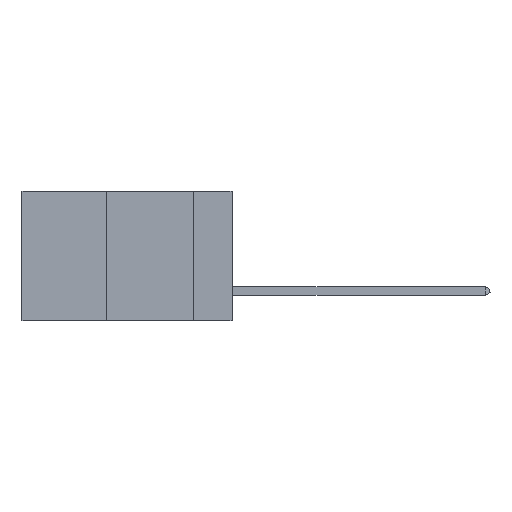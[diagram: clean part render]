
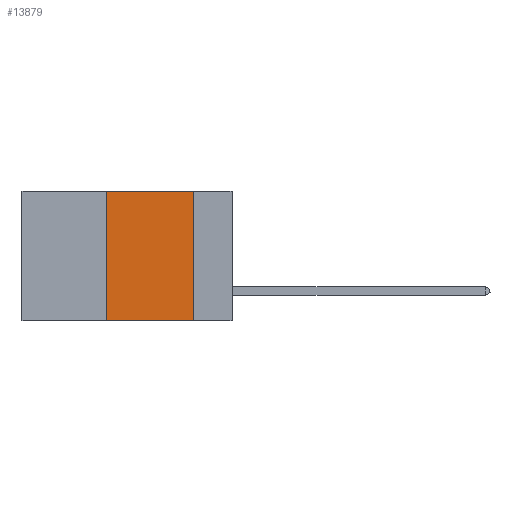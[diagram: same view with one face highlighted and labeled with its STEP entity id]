
A CAD part, left-side view. The second image highlights one B-rep face of the part: STEP entity #13879.
In plain terms, the highlighted planar face has unit normal (-1, 0, 0).
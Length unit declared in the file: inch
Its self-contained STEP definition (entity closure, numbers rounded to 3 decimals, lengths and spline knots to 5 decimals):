
#1645 = EDGE_LOOP ( 'NONE', ( #18609, #4746, #25784, #2938 ) ) ;
#2938 = ORIENTED_EDGE ( 'NONE', *, *, #21262, .T. ) ;
#3064 = DIRECTION ( 'NONE',  ( 0., 0., -1. ) ) ;
#3400 = CARTESIAN_POINT ( 'NONE',  ( 0., 0.36, 0. ) ) ;
#4480 = CARTESIAN_POINT ( 'NONE',  ( 0., 0.6, 0. ) ) ;
#4516 = CARTESIAN_POINT ( 'NONE',  ( 0., 0.11, -0.37 ) ) ;
#4746 = ORIENTED_EDGE ( 'NONE', *, *, #12196, .F. ) ;
#4916 = DIRECTION ( 'NONE',  ( 0., -1., 0. ) ) ;
#5689 = EDGE_CURVE ( 'NONE', #15217, #21051, #22135, .T. ) ;
#6246 = VECTOR ( 'NONE', #3064, 39.37008 ) ;
#6550 = CARTESIAN_POINT ( 'NONE',  ( 0., 0.6, 0. ) ) ;
#6699 = LINE ( 'NONE', #25753, #9295 ) ;
#7883 = EDGE_CURVE ( 'NONE', #17544, #24562, #24001, .T. ) ;
#8630 = DIRECTION ( 'NONE',  ( 0., 0., -1. ) ) ;
#9295 = VECTOR ( 'NONE', #17797, 39.37008 ) ;
#12196 = EDGE_CURVE ( 'NONE', #24562, #15217, #14061, .T. ) ;
#13486 = CARTESIAN_POINT ( 'NONE',  ( 0., 0.11, 0. ) ) ;
#13879 = ADVANCED_FACE ( 'NONE', ( #23405 ), #25015, .F. ) ;
#14061 = LINE ( 'NONE', #4480, #25749 ) ;
#15217 = VERTEX_POINT ( 'NONE', #22149 ) ;
#16197 = AXIS2_PLACEMENT_3D ( 'NONE', #6550, #21054, #8630 ) ;
#16597 = DIRECTION ( 'NONE',  ( 0., 0., 1. ) ) ;
#17526 = CARTESIAN_POINT ( 'NONE',  ( 0., 0.36, -0.37 ) ) ;
#17544 = VERTEX_POINT ( 'NONE', #17526 ) ;
#17797 = DIRECTION ( 'NONE',  ( 0., -1., 0. ) ) ;
#18581 = CARTESIAN_POINT ( 'NONE',  ( 0., 0.36, 0. ) ) ;
#18609 = ORIENTED_EDGE ( 'NONE', *, *, #5689, .F. ) ;
#21051 = VERTEX_POINT ( 'NONE', #4516 ) ;
#21054 = DIRECTION ( 'NONE',  ( 1., 0., 0. ) ) ;
#21262 = EDGE_CURVE ( 'NONE', #17544, #21051, #6699, .T. ) ;
#22135 = LINE ( 'NONE', #13486, #6246 ) ;
#22149 = CARTESIAN_POINT ( 'NONE',  ( 0., 0.11, 0. ) ) ;
#22372 = VECTOR ( 'NONE', #16597, 39.37008 ) ;
#23405 = FACE_OUTER_BOUND ( 'NONE', #1645, .T. ) ;
#24001 = LINE ( 'NONE', #18581, #22372 ) ;
#24562 = VERTEX_POINT ( 'NONE', #3400 ) ;
#25015 = PLANE ( 'NONE',  #16197 ) ;
#25749 = VECTOR ( 'NONE', #4916, 39.37008 ) ;
#25753 = CARTESIAN_POINT ( 'NONE',  ( 0., 0.6, -0.37 ) ) ;
#25784 = ORIENTED_EDGE ( 'NONE', *, *, #7883, .F. ) ;
